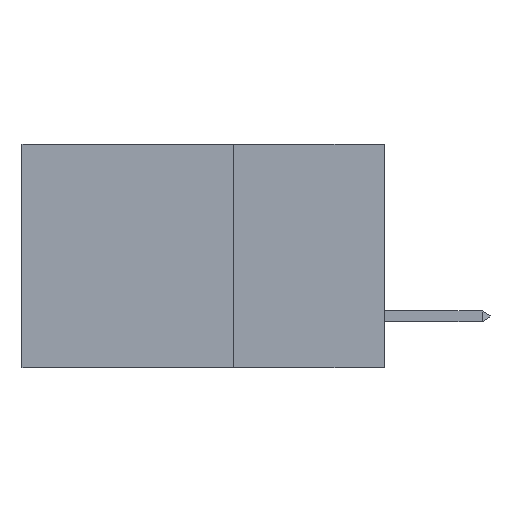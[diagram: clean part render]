
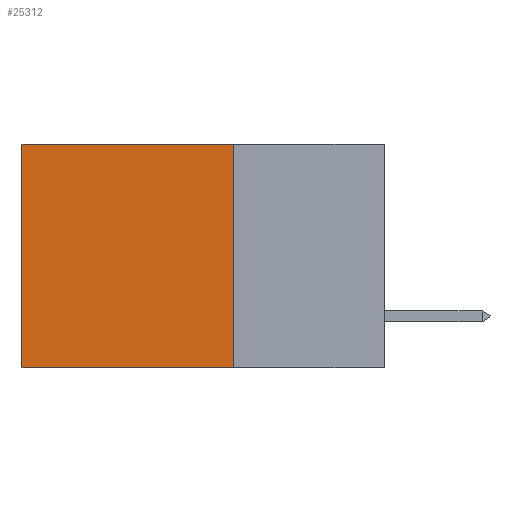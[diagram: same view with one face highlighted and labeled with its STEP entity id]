
A CAD part, left-side view. The second image highlights one B-rep face of the part: STEP entity #25312.
In plain terms, the highlighted planar face has unit normal (-1, 0, 0).
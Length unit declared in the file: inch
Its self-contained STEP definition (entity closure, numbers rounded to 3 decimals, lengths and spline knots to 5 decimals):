
#700 = CARTESIAN_POINT ( 'NONE',  ( 0.2875, 0.6, 0. ) ) ;
#3534 = DIRECTION ( 'NONE',  ( 0., 0., -1. ) ) ;
#3626 = VERTEX_POINT ( 'NONE', #17143 ) ;
#4593 = DIRECTION ( 'NONE',  ( 0., 1., 0. ) ) ;
#8208 = LINE ( 'NONE', #700, #24633 ) ;
#8295 = LINE ( 'NONE', #9259, #24142 ) ;
#9259 = CARTESIAN_POINT ( 'NONE',  ( 0.2875, 0.25, 0. ) ) ;
#10408 = ORIENTED_EDGE ( 'NONE', *, *, #30687, .F. ) ;
#16589 = LINE ( 'NONE', #27614, #46155 ) ;
#17143 = CARTESIAN_POINT ( 'NONE',  ( 0.2875, 0.25, -0.37 ) ) ;
#18172 = CARTESIAN_POINT ( 'NONE',  ( 0.2875, 0.25, 0. ) ) ;
#20672 = VERTEX_POINT ( 'NONE', #48061 ) ;
#20778 = DIRECTION ( 'NONE',  ( 0., 1., 0. ) ) ;
#23344 = LINE ( 'NONE', #41647, #29378 ) ;
#24142 = VECTOR ( 'NONE', #20778, 39.37008 ) ;
#24633 = VECTOR ( 'NONE', #35705, 39.37008 ) ;
#25312 = ADVANCED_FACE ( 'NONE', ( #33315 ), #41095, .F. ) ;
#25622 = CARTESIAN_POINT ( 'NONE',  ( 0.2875, 0.6, -0.37 ) ) ;
#27614 = CARTESIAN_POINT ( 'NONE',  ( 0.2875, 0.25, -0.37 ) ) ;
#29378 = VECTOR ( 'NONE', #34613, 39.37008 ) ;
#30687 = EDGE_CURVE ( 'NONE', #31824, #3626, #23344, .T. ) ;
#31676 = EDGE_CURVE ( 'NONE', #20672, #39223, #8208, .T. ) ;
#31824 = VERTEX_POINT ( 'NONE', #18172 ) ;
#33315 = FACE_OUTER_BOUND ( 'NONE', #48691, .T. ) ;
#34613 = DIRECTION ( 'NONE',  ( 0., 0., -1. ) ) ;
#34770 = ORIENTED_EDGE ( 'NONE', *, *, #31676, .T. ) ;
#35705 = DIRECTION ( 'NONE',  ( 0., 0., -1. ) ) ;
#39219 = ORIENTED_EDGE ( 'NONE', *, *, #46046, .F. ) ;
#39223 = VERTEX_POINT ( 'NONE', #25622 ) ;
#39810 = ORIENTED_EDGE ( 'NONE', *, *, #44192, .T. ) ;
#41095 = PLANE ( 'NONE',  #45802 ) ;
#41647 = CARTESIAN_POINT ( 'NONE',  ( 0.2875, 0.25, 0. ) ) ;
#42074 = DIRECTION ( 'NONE',  ( 1., 0., 0. ) ) ;
#44192 = EDGE_CURVE ( 'NONE', #31824, #20672, #8295, .T. ) ;
#45085 = CARTESIAN_POINT ( 'NONE',  ( 0.2875, 0.25, 0. ) ) ;
#45802 = AXIS2_PLACEMENT_3D ( 'NONE', #45085, #42074, #3534 ) ;
#46046 = EDGE_CURVE ( 'NONE', #3626, #39223, #16589, .T. ) ;
#46155 = VECTOR ( 'NONE', #4593, 39.37008 ) ;
#48061 = CARTESIAN_POINT ( 'NONE',  ( 0.2875, 0.6, 0. ) ) ;
#48691 = EDGE_LOOP ( 'NONE', ( #34770, #39219, #10408, #39810 ) ) ;
